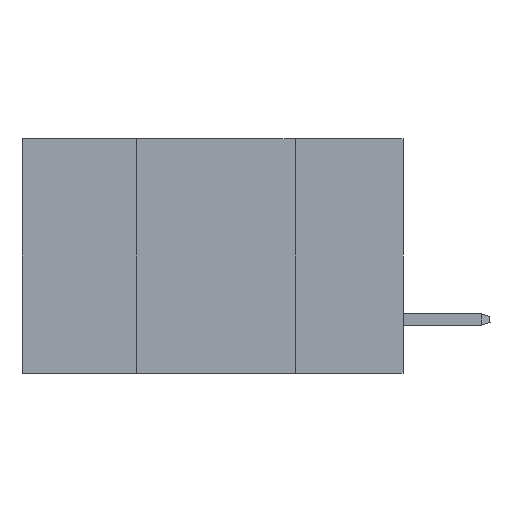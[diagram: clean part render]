
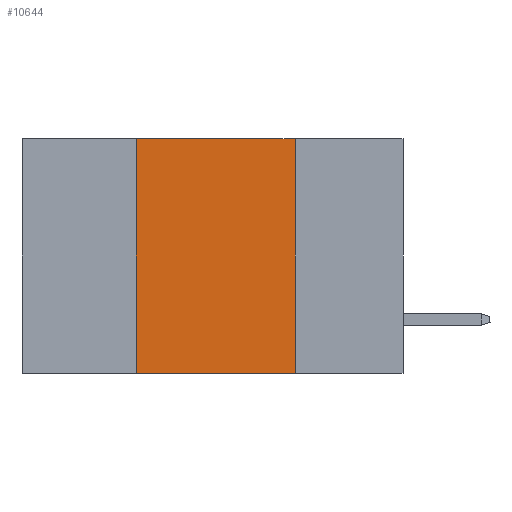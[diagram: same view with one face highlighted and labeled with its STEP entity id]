
A CAD part, left-side view. The second image highlights one B-rep face of the part: STEP entity #10644.
In plain terms, the highlighted planar face has unit normal (-1, 0, 0).
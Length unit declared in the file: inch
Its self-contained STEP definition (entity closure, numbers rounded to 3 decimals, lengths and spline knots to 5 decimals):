
#178 = VERTEX_POINT ( 'NONE', #2337 ) ;
#569 = VECTOR ( 'NONE', #6015, 39.37008 ) ;
#1120 = CARTESIAN_POINT ( 'NONE',  ( 0., 0.6, 0. ) ) ;
#1130 = VERTEX_POINT ( 'NONE', #7522 ) ;
#1840 = DIRECTION ( 'NONE',  ( 0., -1., 0. ) ) ;
#1850 = CARTESIAN_POINT ( 'NONE',  ( 0., 0.17, 0. ) ) ;
#2337 = CARTESIAN_POINT ( 'NONE',  ( 0., 0.42, -0.37 ) ) ;
#3584 = CARTESIAN_POINT ( 'NONE',  ( 0., 0.42, 0. ) ) ;
#5050 = DIRECTION ( 'NONE',  ( 0., 0., -1. ) ) ;
#5229 = EDGE_CURVE ( 'NONE', #178, #1130, #20483, .T. ) ;
#6015 = DIRECTION ( 'NONE',  ( 0., 0., -1. ) ) ;
#7522 = CARTESIAN_POINT ( 'NONE',  ( 0., 0.42, 0. ) ) ;
#9651 = CARTESIAN_POINT ( 'NONE',  ( 0., 0.17, 0. ) ) ;
#9999 = CARTESIAN_POINT ( 'NONE',  ( 0., 0.17, -0.37 ) ) ;
#10644 = ADVANCED_FACE ( 'NONE', ( #20219 ), #18115, .F. ) ;
#10902 = EDGE_LOOP ( 'NONE', ( #22678, #19763, #21814, #15525 ) ) ;
#10986 = VECTOR ( 'NONE', #1840, 39.37008 ) ;
#11084 = DIRECTION ( 'NONE',  ( 0., 0., 1. ) ) ;
#11576 = EDGE_CURVE ( 'NONE', #178, #16616, #12348, .T. ) ;
#11875 = AXIS2_PLACEMENT_3D ( 'NONE', #1120, #14196, #5050 ) ;
#12348 = LINE ( 'NONE', #19875, #14686 ) ;
#13478 = EDGE_CURVE ( 'NONE', #1130, #23595, #18603, .T. ) ;
#14196 = DIRECTION ( 'NONE',  ( 1., 0., 0. ) ) ;
#14658 = CARTESIAN_POINT ( 'NONE',  ( 0., 0.6, 0. ) ) ;
#14686 = VECTOR ( 'NONE', #21615, 39.37008 ) ;
#15525 = ORIENTED_EDGE ( 'NONE', *, *, #11576, .T. ) ;
#16616 = VERTEX_POINT ( 'NONE', #9999 ) ;
#18115 = PLANE ( 'NONE',  #11875 ) ;
#18603 = LINE ( 'NONE', #14658, #10986 ) ;
#18742 = LINE ( 'NONE', #1850, #569 ) ;
#19763 = ORIENTED_EDGE ( 'NONE', *, *, #13478, .F. ) ;
#19875 = CARTESIAN_POINT ( 'NONE',  ( 0., 0.6, -0.37 ) ) ;
#20219 = FACE_OUTER_BOUND ( 'NONE', #10902, .T. ) ;
#20483 = LINE ( 'NONE', #3584, #21639 ) ;
#20801 = EDGE_CURVE ( 'NONE', #23595, #16616, #18742, .T. ) ;
#21615 = DIRECTION ( 'NONE',  ( 0., -1., 0. ) ) ;
#21639 = VECTOR ( 'NONE', #11084, 39.37008 ) ;
#21814 = ORIENTED_EDGE ( 'NONE', *, *, #5229, .F. ) ;
#22678 = ORIENTED_EDGE ( 'NONE', *, *, #20801, .F. ) ;
#23595 = VERTEX_POINT ( 'NONE', #9651 ) ;
